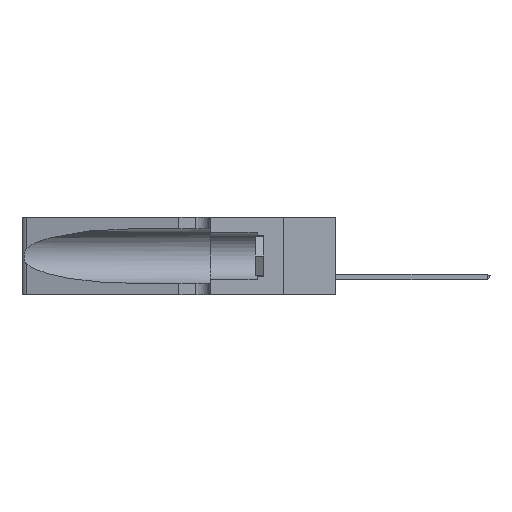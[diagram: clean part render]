
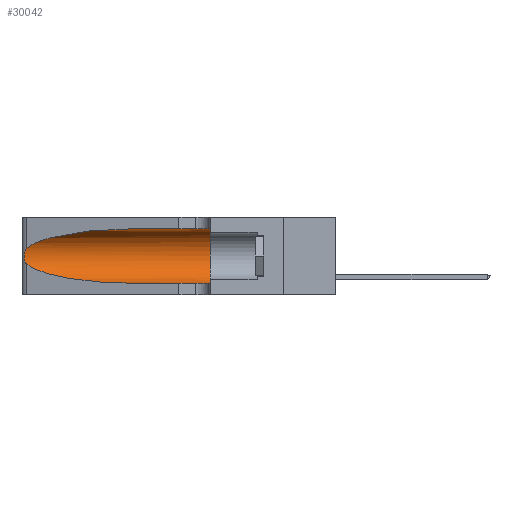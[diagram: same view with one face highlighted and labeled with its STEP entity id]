
A CAD part, left-side view. The second image highlights one B-rep face of the part: STEP entity #30042.
In plain terms, the highlighted cylindrical face has radius 3.308 mm (diameter 6.617 mm), a partial arc.
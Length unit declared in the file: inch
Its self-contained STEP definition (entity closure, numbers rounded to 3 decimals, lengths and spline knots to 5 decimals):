
#540 = ORIENTED_EDGE ( 'NONE', *, *, #10550, .F. ) ;
#715 = CARTESIAN_POINT ( 'NONE',  ( 0.1305, 0.72297, 0.05475 ) ) ;
#1416 = CARTESIAN_POINT ( 'NONE',  ( 0.25487, 1.22718, 0.22369 ) ) ;
#1534 = CARTESIAN_POINT ( 'NONE',  ( 0.1305, 0.35, 0.31525 ) ) ;
#1538 = DIRECTION ( 'NONE',  ( 0., -1., 0. ) ) ;
#1627 = CARTESIAN_POINT ( 'NONE',  ( 0.25487, 1.22718, 0.14631 ) ) ;
#1846 = VERTEX_POINT ( 'NONE', #3378 ) ;
#2166 = LINE ( 'NONE', #12746, #2525 ) ;
#2351 = VERTEX_POINT ( 'NONE', #1416 ) ;
#2525 = VECTOR ( 'NONE', #15172, 39.37008 ) ;
#2544 = AXIS2_PLACEMENT_3D ( 'NONE', #19718, #5529, #5918 ) ;
#3194 = CARTESIAN_POINT ( 'NONE',  ( 0.1305, 0.72297, 0.31525 ) ) ;
#3378 = CARTESIAN_POINT ( 'NONE',  ( 0.1305, 0.72297, 0.05475 ) ) ;
#5529 = DIRECTION ( 'NONE',  ( 0., 1., 0. ) ) ;
#5592 = CARTESIAN_POINT ( 'NONE',  ( 0.2373, 1.15595, 0.08982 ) ) ;
#5876 = ORIENTED_EDGE ( 'NONE', *, *, #25250, .T. ) ;
#5918 = DIRECTION ( 'NONE',  ( 0., 0., 1. ) ) ;
#6203 = VECTOR ( 'NONE', #13956, 39.37008 ) ;
#6339 =( BOUNDED_CURVE ( )  B_SPLINE_CURVE ( 3, ( #18215, #5592, #20770, #715 ),
 .UNSPECIFIED., .F., .T. ) 
 B_SPLINE_CURVE_WITH_KNOTS ( ( 4, 4 ),
 ( 3.44316, 4.71239 ),
 .UNSPECIFIED. ) 
 CURVE ( )  GEOMETRIC_REPRESENTATION_ITEM ( )  RATIONAL_B_SPLINE_CURVE ( ( 1., 0.87, 0.87, 1. ) ) 
 REPRESENTATION_ITEM ( '' )  );
#6505 = CARTESIAN_POINT ( 'NONE',  ( 0.25639, 1.23186, 0.15144 ) ) ;
#7625 = CARTESIAN_POINT ( 'NONE',  ( 0.25787, 1.23484, 0.2124 ) ) ;
#8731 = AXIS2_PLACEMENT_3D ( 'NONE', #13657, #1538, #25994 ) ;
#8873 = LINE ( 'NONE', #14057, #6203 ) ;
#10402 = CARTESIAN_POINT ( 'NONE',  ( 0.25487, 1.22718, 0.14631 ) ) ;
#10550 = EDGE_CURVE ( 'NONE', #31940, #11955, #2166, .T. ) ;
#11768 = CARTESIAN_POINT ( 'NONE',  ( 0.25856, 1.23593, 0.16098 ) ) ;
#11955 = VERTEX_POINT ( 'NONE', #1534 ) ;
#12237 = ORIENTED_EDGE ( 'NONE', *, *, #22661, .T. ) ;
#12592 = EDGE_CURVE ( 'NONE', #11955, #17588, #14756, .T. ) ;
#12746 = CARTESIAN_POINT ( 'NONE',  ( 0.1305, 1.61858, 0.31525 ) ) ;
#13546 = VERTEX_POINT ( 'NONE', #10402 ) ;
#13657 = CARTESIAN_POINT ( 'NONE',  ( 0.1305, 1.61858, 0.185 ) ) ;
#13956 = DIRECTION ( 'NONE',  ( 0., -1., 0. ) ) ;
#14057 = CARTESIAN_POINT ( 'NONE',  ( 0.1305, 1.61858, 0.05475 ) ) ;
#14557 = CARTESIAN_POINT ( 'NONE',  ( 0.25639, 1.23184, 0.21858 ) ) ;
#14756 = CIRCLE ( 'NONE', #2544, 0.13025 ) ;
#15172 = DIRECTION ( 'NONE',  ( 0., -1., 0. ) ) ;
#16603 = CARTESIAN_POINT ( 'NONE',  ( 0.26018, 1.23835, 0.19895 ) ) ;
#17416 = ORIENTED_EDGE ( 'NONE', *, *, #22855, .T. ) ;
#17588 = VERTEX_POINT ( 'NONE', #25249 ) ;
#18215 = CARTESIAN_POINT ( 'NONE',  ( 0.25487, 1.22718, 0.14631 ) ) ;
#19493 = EDGE_CURVE ( 'NONE', #1846, #17588, #8873, .T. ) ;
#19718 = CARTESIAN_POINT ( 'NONE',  ( 0.1305, 0.35, 0.185 ) ) ;
#19989 = CARTESIAN_POINT ( 'NONE',  ( 0.1305, 0.72297, 0.31525 ) ) ;
#20183 = FACE_OUTER_BOUND ( 'NONE', #27737, .T. ) ;
#20524 = CARTESIAN_POINT ( 'NONE',  ( 0.2373, 1.15595, 0.28018 ) ) ;
#20770 = CARTESIAN_POINT ( 'NONE',  ( 0.18966, 0.96281, 0.05475 ) ) ;
#21896 =( BOUNDED_CURVE ( )  B_SPLINE_CURVE ( 3, ( #19989, #27977, #20524, #25465 ),
 .UNSPECIFIED., .F., .F. ) 
 B_SPLINE_CURVE_WITH_KNOTS ( ( 4, 4 ),
 ( 1.5708, 2.84003 ),
 .UNSPECIFIED. ) 
 CURVE ( )  GEOMETRIC_REPRESENTATION_ITEM ( )  RATIONAL_B_SPLINE_CURVE ( ( 1., 0.87, 0.87, 1. ) ) 
 REPRESENTATION_ITEM ( '' )  );
#22661 = EDGE_CURVE ( 'NONE', #2351, #13546, #29220, .T. ) ;
#22855 = EDGE_CURVE ( 'NONE', #31940, #2351, #21896, .T. ) ;
#23794 = CARTESIAN_POINT ( 'NONE',  ( 0.26075, 1.23896, 0.178 ) ) ;
#24011 = CARTESIAN_POINT ( 'NONE',  ( 0.26075, 1.23896, 0.19203 ) ) ;
#24115 = CARTESIAN_POINT ( 'NONE',  ( 0.25487, 1.22718, 0.22369 ) ) ;
#24809 = CYLINDRICAL_SURFACE ( 'NONE', #8731, 0.13025 ) ;
#25027 = ORIENTED_EDGE ( 'NONE', *, *, #12592, .F. ) ;
#25138 = CARTESIAN_POINT ( 'NONE',  ( 0.25854, 1.2359, 0.20912 ) ) ;
#25249 = CARTESIAN_POINT ( 'NONE',  ( 0.1305, 0.35, 0.05475 ) ) ;
#25250 = EDGE_CURVE ( 'NONE', #13546, #1846, #6339, .T. ) ;
#25465 = CARTESIAN_POINT ( 'NONE',  ( 0.25487, 1.22718, 0.22369 ) ) ;
#25994 = DIRECTION ( 'NONE',  ( 0., 0., -1. ) ) ;
#26485 = CARTESIAN_POINT ( 'NONE',  ( 0.26017, 1.23833, 0.17102 ) ) ;
#27548 = ORIENTED_EDGE ( 'NONE', *, *, #19493, .T. ) ;
#27737 = EDGE_LOOP ( 'NONE', ( #17416, #12237, #5876, #27548, #25027, #540 ) ) ;
#27977 = CARTESIAN_POINT ( 'NONE',  ( 0.18966, 0.96281, 0.31525 ) ) ;
#28382 = CARTESIAN_POINT ( 'NONE',  ( 0.25555, 1.22994, 0.2215 ) ) ;
#28567 = CARTESIAN_POINT ( 'NONE',  ( 0.25789, 1.23486, 0.15765 ) ) ;
#29220 = B_SPLINE_CURVE_WITH_KNOTS ( 'NONE', 3,
 ( #24115, #28382, #14557, #7625, #25138, #16603, #24011, #23794, #26485, #11768, #28567, #6505, #31125, #1627 ),
 .UNSPECIFIED., .F., .F.,
 ( 4, 2, 2, 2, 2, 2, 4 ),
 ( 0., 0.00027, 0.00053, 0.00107, 0.0016, 0.00187, 0.00214 ),
 .UNSPECIFIED. ) ;
#30042 = ADVANCED_FACE ( 'NONE', ( #20183 ), #24809, .F. ) ;
#31125 = CARTESIAN_POINT ( 'NONE',  ( 0.25555, 1.22993, 0.14849 ) ) ;
#31940 = VERTEX_POINT ( 'NONE', #3194 ) ;
